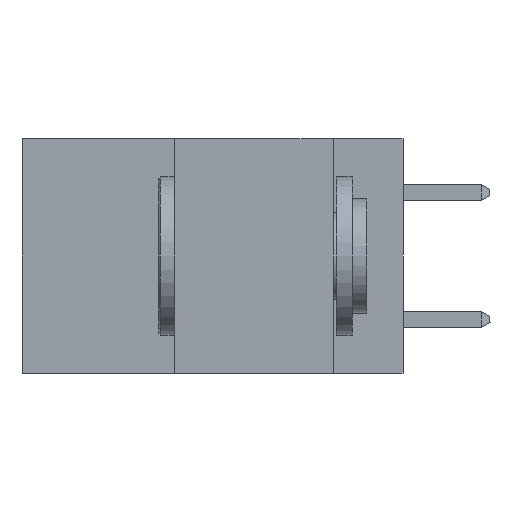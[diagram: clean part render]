
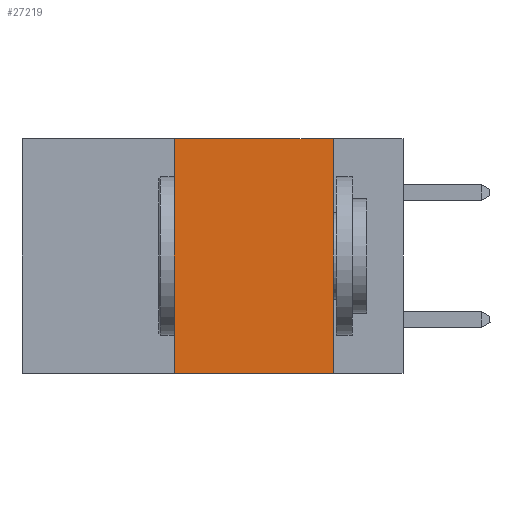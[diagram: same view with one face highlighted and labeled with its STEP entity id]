
A CAD part, left-side view. The second image highlights one B-rep face of the part: STEP entity #27219.
In plain terms, the highlighted planar face has unit normal (-1, 0, 0).
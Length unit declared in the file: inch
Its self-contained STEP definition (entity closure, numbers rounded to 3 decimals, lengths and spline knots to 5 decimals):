
#241 = LINE ( 'NONE', #17675, #12540 ) ;
#1159 = ORIENTED_EDGE ( 'NONE', *, *, #9957, .F. ) ;
#1944 = ORIENTED_EDGE ( 'NONE', *, *, #22673, .F. ) ;
#2272 = FACE_OUTER_BOUND ( 'NONE', #7295, .T. ) ;
#3277 = EDGE_CURVE ( 'NONE', #9662, #22688, #20976, .T. ) ;
#4343 = DIRECTION ( 'NONE',  ( 1., 0., 0. ) ) ;
#6254 = CARTESIAN_POINT ( 'NONE',  ( 0., 0.11, 0. ) ) ;
#7295 = EDGE_LOOP ( 'NONE', ( #1944, #13006, #1159, #29027 ) ) ;
#8251 = VERTEX_POINT ( 'NONE', #17365 ) ;
#8867 = VECTOR ( 'NONE', #13731, 39.37008 ) ;
#9662 = VERTEX_POINT ( 'NONE', #17819 ) ;
#9957 = EDGE_CURVE ( 'NONE', #9662, #8251, #16131, .T. ) ;
#12540 = VECTOR ( 'NONE', #17471, 39.37008 ) ;
#13006 = ORIENTED_EDGE ( 'NONE', *, *, #19652, .F. ) ;
#13129 = CARTESIAN_POINT ( 'NONE',  ( 0., 0.11, -0.37 ) ) ;
#13661 = CARTESIAN_POINT ( 'NONE',  ( 0., 0.6, 0. ) ) ;
#13731 = DIRECTION ( 'NONE',  ( 0., 0., 1. ) ) ;
#13888 = VERTEX_POINT ( 'NONE', #6254 ) ;
#14477 = VECTOR ( 'NONE', #26342, 39.37008 ) ;
#16131 = LINE ( 'NONE', #23371, #8867 ) ;
#16496 = VECTOR ( 'NONE', #23622, 39.37008 ) ;
#16509 = CARTESIAN_POINT ( 'NONE',  ( 0., 0.6, 0. ) ) ;
#17365 = CARTESIAN_POINT ( 'NONE',  ( 0., 0.36, 0. ) ) ;
#17471 = DIRECTION ( 'NONE',  ( 0., 0., -1. ) ) ;
#17675 = CARTESIAN_POINT ( 'NONE',  ( 0., 0.11, 0. ) ) ;
#17819 = CARTESIAN_POINT ( 'NONE',  ( 0., 0.36, -0.37 ) ) ;
#19652 = EDGE_CURVE ( 'NONE', #8251, #13888, #29637, .T. ) ;
#20976 = LINE ( 'NONE', #28527, #14477 ) ;
#22673 = EDGE_CURVE ( 'NONE', #13888, #22688, #241, .T. ) ;
#22688 = VERTEX_POINT ( 'NONE', #13129 ) ;
#23371 = CARTESIAN_POINT ( 'NONE',  ( 0., 0.36, 0. ) ) ;
#23622 = DIRECTION ( 'NONE',  ( 0., -1., 0. ) ) ;
#23741 = DIRECTION ( 'NONE',  ( 0., 0., -1. ) ) ;
#26342 = DIRECTION ( 'NONE',  ( 0., -1., 0. ) ) ;
#27219 = ADVANCED_FACE ( 'NONE', ( #2272 ), #28303, .F. ) ;
#28303 = PLANE ( 'NONE',  #30413 ) ;
#28527 = CARTESIAN_POINT ( 'NONE',  ( 0., 0.6, -0.37 ) ) ;
#29027 = ORIENTED_EDGE ( 'NONE', *, *, #3277, .T. ) ;
#29637 = LINE ( 'NONE', #16509, #16496 ) ;
#30413 = AXIS2_PLACEMENT_3D ( 'NONE', #13661, #4343, #23741 ) ;
